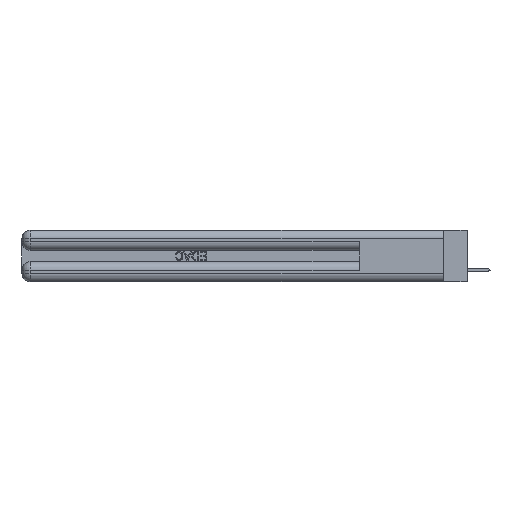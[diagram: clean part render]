
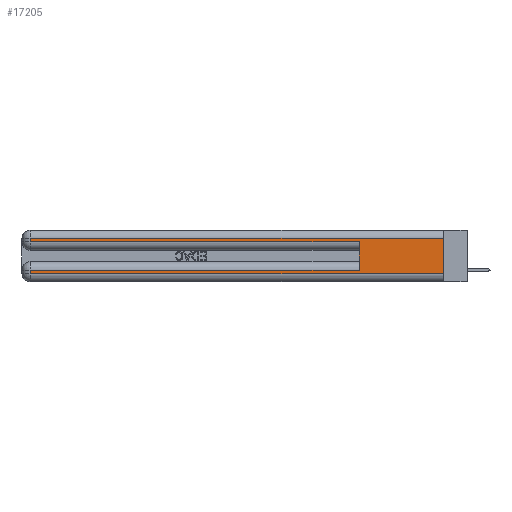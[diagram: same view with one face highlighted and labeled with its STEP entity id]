
A CAD part, left-side view. The second image highlights one B-rep face of the part: STEP entity #17205.
In plain terms, the highlighted planar face has unit normal (-1, 0, 0).
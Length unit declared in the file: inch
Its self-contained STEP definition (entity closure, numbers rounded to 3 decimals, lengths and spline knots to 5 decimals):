
#23 = ORIENTED_EDGE ( 'NONE', *, *, #36019, .T. ) ;
#947 = CARTESIAN_POINT ( 'NONE',  ( 0., 0.6, 0.285 ) ) ;
#1041 = VERTEX_POINT ( 'NONE', #1249 ) ;
#1249 = CARTESIAN_POINT ( 'NONE',  ( 0., 0.6, 0.085 ) ) ;
#3694 = ORIENTED_EDGE ( 'NONE', *, *, #29516, .F. ) ;
#4163 = ORIENTED_EDGE ( 'NONE', *, *, #15374, .F. ) ;
#7215 = ORIENTED_EDGE ( 'NONE', *, *, #19211, .T. ) ;
#8119 = LINE ( 'NONE', #28256, #23654 ) ;
#9139 = VERTEX_POINT ( 'NONE', #18799 ) ;
#10724 = LINE ( 'NONE', #31144, #35164 ) ;
#11326 = VERTEX_POINT ( 'NONE', #33732 ) ;
#12548 = DIRECTION ( 'NONE',  ( 0., 0., -1. ) ) ;
#13258 = VERTEX_POINT ( 'NONE', #26892 ) ;
#13476 = VERTEX_POINT ( 'NONE', #34067 ) ;
#13727 = DIRECTION ( 'NONE',  ( 1., 0., 0. ) ) ;
#14370 = VECTOR ( 'NONE', #19672, 39.37008 ) ;
#14765 = DIRECTION ( 'NONE',  ( 0., 0., -1. ) ) ;
#15187 = DIRECTION ( 'NONE',  ( 0., -1., 0. ) ) ;
#15374 = EDGE_CURVE ( 'NONE', #1041, #20039, #8119, .T. ) ;
#15784 = LINE ( 'NONE', #36683, #24216 ) ;
#17205 = ADVANCED_FACE ( 'NONE', ( #35698 ), #26200, .F. ) ;
#18630 = DIRECTION ( 'NONE',  ( 0., -1., 0. ) ) ;
#18799 = CARTESIAN_POINT ( 'NONE',  ( 0., 2.94, 0.285 ) ) ;
#18812 = LINE ( 'NONE', #36014, #30083 ) ;
#19211 = EDGE_CURVE ( 'NONE', #30237, #38109, #15784, .T. ) ;
#19586 = EDGE_CURVE ( 'NONE', #1041, #13258, #26613, .T. ) ;
#19672 = DIRECTION ( 'NONE',  ( 0., 0., -1. ) ) ;
#20039 = VERTEX_POINT ( 'NONE', #947 ) ;
#21121 = DIRECTION ( 'NONE',  ( 0., 1., 0. ) ) ;
#21440 = DIRECTION ( 'NONE',  ( 0., 1., 0. ) ) ;
#21619 = CARTESIAN_POINT ( 'NONE',  ( 0., 2.94, 0.37 ) ) ;
#22325 = LINE ( 'NONE', #38145, #14370 ) ;
#22754 = EDGE_LOOP ( 'NONE', ( #3694, #36722, #33147, #23, #4163, #29013, #37267, #7215 ) ) ;
#23141 = CARTESIAN_POINT ( 'NONE',  ( 0., 0., 0.085 ) ) ;
#23412 = EDGE_CURVE ( 'NONE', #13258, #30237, #32073, .T. ) ;
#23641 = VECTOR ( 'NONE', #36555, 39.37008 ) ;
#23654 = VECTOR ( 'NONE', #27859, 39.37008 ) ;
#23892 = EDGE_CURVE ( 'NONE', #11326, #13476, #18812, .T. ) ;
#24216 = VECTOR ( 'NONE', #15187, 39.37008 ) ;
#26200 = PLANE ( 'NONE',  #38407 ) ;
#26613 = LINE ( 'NONE', #23141, #28977 ) ;
#26892 = CARTESIAN_POINT ( 'NONE',  ( 0., 2.94, 0.085 ) ) ;
#27837 = CARTESIAN_POINT ( 'NONE',  ( 0., 0., 0.37 ) ) ;
#27859 = DIRECTION ( 'NONE',  ( 0., 0., 1. ) ) ;
#28256 = CARTESIAN_POINT ( 'NONE',  ( 0., 0.6, 0.145 ) ) ;
#28319 = VECTOR ( 'NONE', #12548, 39.37008 ) ;
#28378 = EDGE_CURVE ( 'NONE', #13476, #9139, #22325, .T. ) ;
#28977 = VECTOR ( 'NONE', #21121, 39.37008 ) ;
#28995 = CARTESIAN_POINT ( 'NONE',  ( 0., 0., 0.06 ) ) ;
#29013 = ORIENTED_EDGE ( 'NONE', *, *, #19586, .T. ) ;
#29516 = EDGE_CURVE ( 'NONE', #11326, #38109, #31653, .T. ) ;
#30083 = VECTOR ( 'NONE', #21440, 39.37008 ) ;
#30237 = VERTEX_POINT ( 'NONE', #30500 ) ;
#30500 = CARTESIAN_POINT ( 'NONE',  ( 0., 2.94, 0.06 ) ) ;
#31144 = CARTESIAN_POINT ( 'NONE',  ( 0., 0., 0.285 ) ) ;
#31653 = LINE ( 'NONE', #27837, #23641 ) ;
#32073 = LINE ( 'NONE', #21619, #28319 ) ;
#33147 = ORIENTED_EDGE ( 'NONE', *, *, #28378, .T. ) ;
#33732 = CARTESIAN_POINT ( 'NONE',  ( 0., 0., 0.31 ) ) ;
#34067 = CARTESIAN_POINT ( 'NONE',  ( 0., 2.94, 0.31 ) ) ;
#35164 = VECTOR ( 'NONE', #18630, 39.37008 ) ;
#35698 = FACE_OUTER_BOUND ( 'NONE', #22754, .T. ) ;
#36014 = CARTESIAN_POINT ( 'NONE',  ( 0., 0., 0.31 ) ) ;
#36019 = EDGE_CURVE ( 'NONE', #9139, #20039, #10724, .T. ) ;
#36555 = DIRECTION ( 'NONE',  ( 0., 0., -1. ) ) ;
#36683 = CARTESIAN_POINT ( 'NONE',  ( 0., 0., 0.06 ) ) ;
#36722 = ORIENTED_EDGE ( 'NONE', *, *, #23892, .T. ) ;
#37267 = ORIENTED_EDGE ( 'NONE', *, *, #23412, .T. ) ;
#37620 = CARTESIAN_POINT ( 'NONE',  ( 0., 0., 0.37 ) ) ;
#38109 = VERTEX_POINT ( 'NONE', #28995 ) ;
#38145 = CARTESIAN_POINT ( 'NONE',  ( 0., 2.94, 0.37 ) ) ;
#38407 = AXIS2_PLACEMENT_3D ( 'NONE', #37620, #13727, #14765 ) ;
